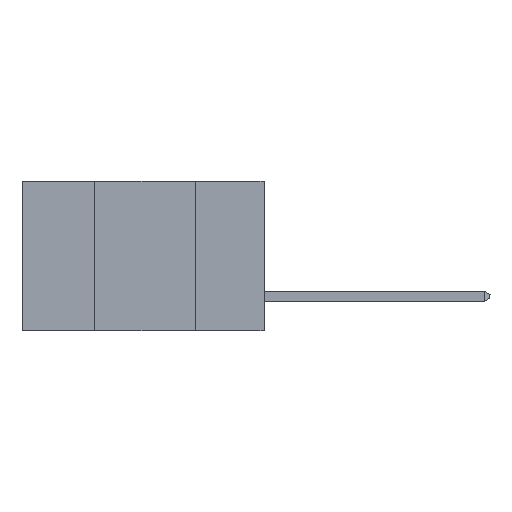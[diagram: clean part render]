
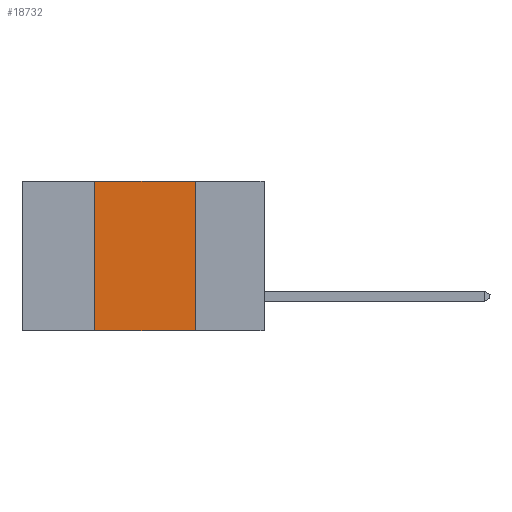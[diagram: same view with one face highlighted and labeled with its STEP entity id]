
A CAD part, left-side view. The second image highlights one B-rep face of the part: STEP entity #18732.
In plain terms, the highlighted planar face has unit normal (-1, 0, 0).
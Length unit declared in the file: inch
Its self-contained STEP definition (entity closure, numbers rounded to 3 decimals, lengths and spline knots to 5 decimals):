
#990 = CARTESIAN_POINT ( 'NONE',  ( 0., 0.6, 0. ) ) ;
#1811 = AXIS2_PLACEMENT_3D ( 'NONE', #990, #14009, #12023 ) ;
#2867 = CARTESIAN_POINT ( 'NONE',  ( 0., 0.42, 0. ) ) ;
#3870 = VERTEX_POINT ( 'NONE', #19326 ) ;
#4363 = DIRECTION ( 'NONE',  ( 0., -1., 0. ) ) ;
#4582 = VERTEX_POINT ( 'NONE', #18784 ) ;
#5155 = VECTOR ( 'NONE', #16632, 39.37008 ) ;
#6880 = EDGE_CURVE ( 'NONE', #4582, #21822, #7721, .T. ) ;
#7721 = LINE ( 'NONE', #19715, #5155 ) ;
#9016 = VECTOR ( 'NONE', #19181, 39.37008 ) ;
#9103 = EDGE_CURVE ( 'NONE', #3870, #21822, #9765, .T. ) ;
#9765 = LINE ( 'NONE', #11755, #20571 ) ;
#9869 = EDGE_CURVE ( 'NONE', #3870, #14931, #12902, .T. ) ;
#9904 = CARTESIAN_POINT ( 'NONE',  ( 0., 0.6, 0. ) ) ;
#9905 = FACE_OUTER_BOUND ( 'NONE', #15539, .T. ) ;
#10618 = CARTESIAN_POINT ( 'NONE',  ( 0., 0.17, -0.37 ) ) ;
#11124 = CARTESIAN_POINT ( 'NONE',  ( 0., 0.42, -0.37 ) ) ;
#11755 = CARTESIAN_POINT ( 'NONE',  ( 0., 0.6, -0.37 ) ) ;
#12023 = DIRECTION ( 'NONE',  ( 0., 0., -1. ) ) ;
#12159 = ORIENTED_EDGE ( 'NONE', *, *, #9103, .T. ) ;
#12277 = EDGE_CURVE ( 'NONE', #14931, #4582, #13775, .T. ) ;
#12551 = ORIENTED_EDGE ( 'NONE', *, *, #6880, .F. ) ;
#12902 = LINE ( 'NONE', #11124, #13872 ) ;
#13775 = LINE ( 'NONE', #9904, #9016 ) ;
#13872 = VECTOR ( 'NONE', #14534, 39.37008 ) ;
#14009 = DIRECTION ( 'NONE',  ( 1., 0., 0. ) ) ;
#14383 = ORIENTED_EDGE ( 'NONE', *, *, #9869, .F. ) ;
#14534 = DIRECTION ( 'NONE',  ( 0., 0., 1. ) ) ;
#14931 = VERTEX_POINT ( 'NONE', #2867 ) ;
#15539 = EDGE_LOOP ( 'NONE', ( #12551, #21949, #14383, #12159 ) ) ;
#16632 = DIRECTION ( 'NONE',  ( 0., 0., -1. ) ) ;
#17062 = PLANE ( 'NONE',  #1811 ) ;
#18732 = ADVANCED_FACE ( 'NONE', ( #9905 ), #17062, .F. ) ;
#18784 = CARTESIAN_POINT ( 'NONE',  ( 0., 0.17, 0. ) ) ;
#19181 = DIRECTION ( 'NONE',  ( 0., -1., 0. ) ) ;
#19326 = CARTESIAN_POINT ( 'NONE',  ( 0., 0.42, -0.37 ) ) ;
#19715 = CARTESIAN_POINT ( 'NONE',  ( 0., 0.17, -0.37 ) ) ;
#20571 = VECTOR ( 'NONE', #4363, 39.37008 ) ;
#21822 = VERTEX_POINT ( 'NONE', #10618 ) ;
#21949 = ORIENTED_EDGE ( 'NONE', *, *, #12277, .F. ) ;
